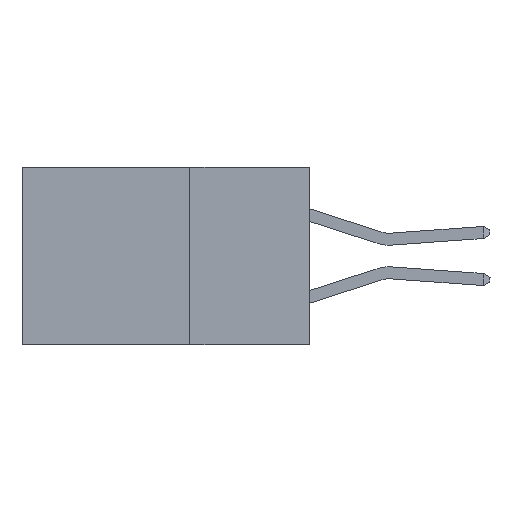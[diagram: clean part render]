
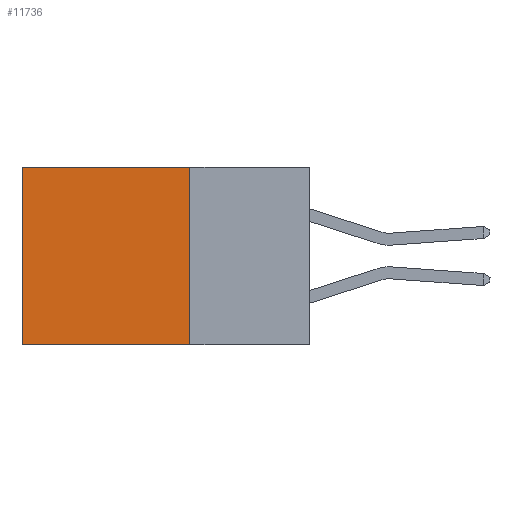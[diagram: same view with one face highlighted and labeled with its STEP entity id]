
A CAD part, left-side view. The second image highlights one B-rep face of the part: STEP entity #11736.
In plain terms, the highlighted planar face has unit normal (-1, 0, 0).
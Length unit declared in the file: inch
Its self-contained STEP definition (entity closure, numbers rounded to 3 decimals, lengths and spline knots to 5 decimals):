
#926 = LINE ( 'NONE', #2404, #9354 ) ;
#1067 = CARTESIAN_POINT ( 'NONE',  ( 0.298, 0.25, 0. ) ) ;
#1185 = EDGE_LOOP ( 'NONE', ( #2112, #1341, #6871, #5212 ) ) ;
#1341 = ORIENTED_EDGE ( 'NONE', *, *, #6315, .F. ) ;
#2112 = ORIENTED_EDGE ( 'NONE', *, *, #6917, .T. ) ;
#2404 = CARTESIAN_POINT ( 'NONE',  ( 0.298, 0.25, -0.37 ) ) ;
#2545 = DIRECTION ( 'NONE',  ( 0., 1., 0. ) ) ;
#3408 = LINE ( 'NONE', #1067, #5325 ) ;
#4714 = VERTEX_POINT ( 'NONE', #13597 ) ;
#5212 = ORIENTED_EDGE ( 'NONE', *, *, #10051, .T. ) ;
#5325 = VECTOR ( 'NONE', #13460, 39.37008 ) ;
#5403 = CARTESIAN_POINT ( 'NONE',  ( 0.298, 0.25, 0. ) ) ;
#6315 = EDGE_CURVE ( 'NONE', #4714, #7977, #926, .T. ) ;
#6611 = CARTESIAN_POINT ( 'NONE',  ( 0.298, 0.6, 0. ) ) ;
#6683 = PLANE ( 'NONE',  #10784 ) ;
#6871 = ORIENTED_EDGE ( 'NONE', *, *, #13828, .F. ) ;
#6917 = EDGE_CURVE ( 'NONE', #12942, #7977, #7409, .T. ) ;
#6919 = CARTESIAN_POINT ( 'NONE',  ( 0.298, 0.25, 0. ) ) ;
#6927 = VERTEX_POINT ( 'NONE', #11665 ) ;
#7409 = LINE ( 'NONE', #10385, #8988 ) ;
#7482 = VECTOR ( 'NONE', #10326, 39.37008 ) ;
#7977 = VERTEX_POINT ( 'NONE', #10110 ) ;
#8988 = VECTOR ( 'NONE', #11517, 39.37008 ) ;
#9354 = VECTOR ( 'NONE', #2545, 39.37008 ) ;
#10051 = EDGE_CURVE ( 'NONE', #6927, #12942, #12415, .T. ) ;
#10110 = CARTESIAN_POINT ( 'NONE',  ( 0.298, 0.6, -0.37 ) ) ;
#10326 = DIRECTION ( 'NONE',  ( 0., 1., 0. ) ) ;
#10385 = CARTESIAN_POINT ( 'NONE',  ( 0.298, 0.6, 0. ) ) ;
#10784 = AXIS2_PLACEMENT_3D ( 'NONE', #5403, #13307, #14400 ) ;
#11517 = DIRECTION ( 'NONE',  ( 0., 0., -1. ) ) ;
#11665 = CARTESIAN_POINT ( 'NONE',  ( 0.298, 0.25, 0. ) ) ;
#11736 = ADVANCED_FACE ( 'NONE', ( #12458 ), #6683, .F. ) ;
#12415 = LINE ( 'NONE', #6919, #7482 ) ;
#12458 = FACE_OUTER_BOUND ( 'NONE', #1185, .T. ) ;
#12942 = VERTEX_POINT ( 'NONE', #6611 ) ;
#13307 = DIRECTION ( 'NONE',  ( 1., 0., 0. ) ) ;
#13460 = DIRECTION ( 'NONE',  ( 0., 0., -1. ) ) ;
#13597 = CARTESIAN_POINT ( 'NONE',  ( 0.298, 0.25, -0.37 ) ) ;
#13828 = EDGE_CURVE ( 'NONE', #6927, #4714, #3408, .T. ) ;
#14400 = DIRECTION ( 'NONE',  ( 0., 0., -1. ) ) ;
